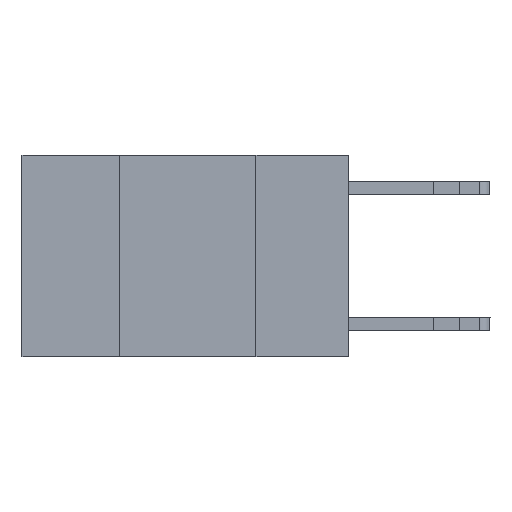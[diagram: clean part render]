
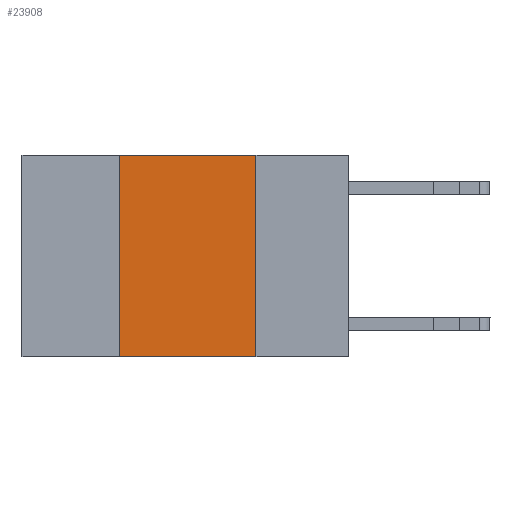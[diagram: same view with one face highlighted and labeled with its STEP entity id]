
A CAD part, left-side view. The second image highlights one B-rep face of the part: STEP entity #23908.
In plain terms, the highlighted planar face has unit normal (-1, 0, 0).
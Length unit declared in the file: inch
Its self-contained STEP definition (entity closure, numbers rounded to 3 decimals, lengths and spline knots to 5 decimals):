
#137 = CARTESIAN_POINT ( 'NONE',  ( 0., 0.6, -0.37 ) ) ;
#1952 = EDGE_LOOP ( 'NONE', ( #3395, #7383, #7051, #6752 ) ) ;
#2019 = DIRECTION ( 'NONE',  ( 0., 0., -1. ) ) ;
#2023 = CARTESIAN_POINT ( 'NONE',  ( 0., 0.17, 0. ) ) ;
#2080 = CARTESIAN_POINT ( 'NONE',  ( 0., 0.42, 0. ) ) ;
#3053 = CARTESIAN_POINT ( 'NONE',  ( 0., 0.42, -0.37 ) ) ;
#3395 = ORIENTED_EDGE ( 'NONE', *, *, #3584, .F. ) ;
#3584 = EDGE_CURVE ( 'NONE', #21173, #24315, #20610, .T. ) ;
#3782 = VECTOR ( 'NONE', #7045, 39.37008 ) ;
#3943 = LINE ( 'NONE', #7020, #3782 ) ;
#4358 = CARTESIAN_POINT ( 'NONE',  ( 0., 0.42, 0. ) ) ;
#4682 = PLANE ( 'NONE',  #12768 ) ;
#5260 = EDGE_CURVE ( 'NONE', #24278, #21173, #3943, .T. ) ;
#6230 = CARTESIAN_POINT ( 'NONE',  ( 0., 0.17, -0.37 ) ) ;
#6251 = DIRECTION ( 'NONE',  ( 0., -1., 0. ) ) ;
#6513 = CARTESIAN_POINT ( 'NONE',  ( 0., 0.17, 0. ) ) ;
#6684 = DIRECTION ( 'NONE',  ( 1., 0., 0. ) ) ;
#6752 = ORIENTED_EDGE ( 'NONE', *, *, #17574, .T. ) ;
#7020 = CARTESIAN_POINT ( 'NONE',  ( 0., 0.6, 0. ) ) ;
#7045 = DIRECTION ( 'NONE',  ( 0., -1., 0. ) ) ;
#7051 = ORIENTED_EDGE ( 'NONE', *, *, #15503, .F. ) ;
#7383 = ORIENTED_EDGE ( 'NONE', *, *, #5260, .F. ) ;
#8278 = VECTOR ( 'NONE', #21916, 39.37008 ) ;
#8334 = LINE ( 'NONE', #4358, #8278 ) ;
#12768 = AXIS2_PLACEMENT_3D ( 'NONE', #18433, #6684, #20332 ) ;
#15498 = FACE_OUTER_BOUND ( 'NONE', #1952, .T. ) ;
#15503 = EDGE_CURVE ( 'NONE', #25170, #24278, #8334, .T. ) ;
#17574 = EDGE_CURVE ( 'NONE', #25170, #24315, #21166, .T. ) ;
#18433 = CARTESIAN_POINT ( 'NONE',  ( 0., 0.6, 0. ) ) ;
#19978 = VECTOR ( 'NONE', #2019, 39.37008 ) ;
#20332 = DIRECTION ( 'NONE',  ( 0., 0., -1. ) ) ;
#20610 = LINE ( 'NONE', #2023, #19978 ) ;
#20738 = VECTOR ( 'NONE', #6251, 39.37008 ) ;
#21166 = LINE ( 'NONE', #137, #20738 ) ;
#21173 = VERTEX_POINT ( 'NONE', #6513 ) ;
#21916 = DIRECTION ( 'NONE',  ( 0., 0., 1. ) ) ;
#23908 = ADVANCED_FACE ( 'NONE', ( #15498 ), #4682, .F. ) ;
#24278 = VERTEX_POINT ( 'NONE', #2080 ) ;
#24315 = VERTEX_POINT ( 'NONE', #6230 ) ;
#25170 = VERTEX_POINT ( 'NONE', #3053 ) ;
